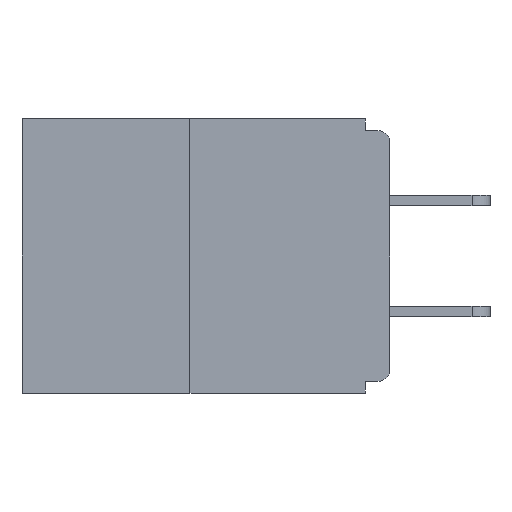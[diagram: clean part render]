
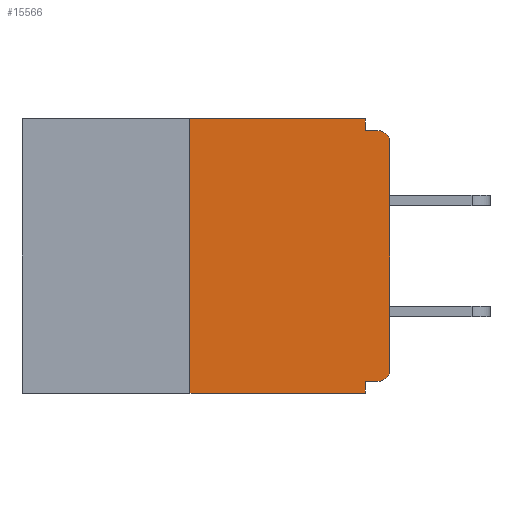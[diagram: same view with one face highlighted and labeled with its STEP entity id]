
A CAD part, left-side view. The second image highlights one B-rep face of the part: STEP entity #15566.
In plain terms, the highlighted planar face has unit normal (-1, 0, 0).
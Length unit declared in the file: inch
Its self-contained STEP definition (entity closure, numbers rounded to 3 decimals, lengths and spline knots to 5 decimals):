
#357 = VERTEX_POINT ( 'NONE', #9742 ) ;
#506 = VECTOR ( 'NONE', #11299, 39.37008 ) ;
#671 = DIRECTION ( 'NONE',  ( 0., 0., 1. ) ) ;
#675 = VECTOR ( 'NONE', #4739, 39.37008 ) ;
#693 = AXIS2_PLACEMENT_3D ( 'NONE', #9688, #7070, #15777 ) ;
#723 = VERTEX_POINT ( 'NONE', #13033 ) ;
#796 = AXIS2_PLACEMENT_3D ( 'NONE', #6944, #5755, #15402 ) ;
#924 = VERTEX_POINT ( 'NONE', #9334 ) ;
#1156 = EDGE_LOOP ( 'NONE', ( #6539, #14464, #13725, #7152, #11252, #13075, #14799, #13834, #2690, #3766 ) ) ;
#1296 = CARTESIAN_POINT ( 'NONE',  ( 0., 0.031, 0. ) ) ;
#1321 = CARTESIAN_POINT ( 'NONE',  ( 0., 0.031, -0.343 ) ) ;
#1667 = DIRECTION ( 'NONE',  ( 0., 0., -1. ) ) ;
#2594 = LINE ( 'NONE', #12889, #14806 ) ;
#2690 = ORIENTED_EDGE ( 'NONE', *, *, #5929, .F. ) ;
#2918 = VERTEX_POINT ( 'NONE', #1321 ) ;
#3150 = DIRECTION ( 'NONE',  ( 0., 0., 1. ) ) ;
#3162 = DIRECTION ( 'NONE',  ( 0., 1., 0. ) ) ;
#3386 = CARTESIAN_POINT ( 'NONE',  ( 0., 0.46, 0. ) ) ;
#3417 = VERTEX_POINT ( 'NONE', #5315 ) ;
#3766 = ORIENTED_EDGE ( 'NONE', *, *, #11858, .F. ) ;
#3894 = CIRCLE ( 'NONE', #693, 0.015 ) ;
#4316 = CARTESIAN_POINT ( 'NONE',  ( 0., 0.031, -0.343 ) ) ;
#4546 = EDGE_CURVE ( 'NONE', #723, #13877, #11496, .T. ) ;
#4739 = DIRECTION ( 'NONE',  ( 0., -1., 0. ) ) ;
#4952 = CIRCLE ( 'NONE', #9415, 0.015 ) ;
#5315 = CARTESIAN_POINT ( 'NONE',  ( 0., 0.031, -0.015 ) ) ;
#5355 = LINE ( 'NONE', #1296, #13733 ) ;
#5410 = EDGE_CURVE ( 'NONE', #14856, #723, #4952, .T. ) ;
#5696 = LINE ( 'NONE', #11544, #9718 ) ;
#5755 = DIRECTION ( 'NONE',  ( 1., 0., 0. ) ) ;
#5929 = EDGE_CURVE ( 'NONE', #3417, #924, #5696, .T. ) ;
#6289 = DIRECTION ( 'NONE',  ( 0., 0., -1. ) ) ;
#6325 = CARTESIAN_POINT ( 'NONE',  ( 0., 0.25, 0. ) ) ;
#6335 = CARTESIAN_POINT ( 'NONE',  ( 0., 0.46, -0.343 ) ) ;
#6442 = DIRECTION ( 'NONE',  ( -1., 0., 0. ) ) ;
#6539 = ORIENTED_EDGE ( 'NONE', *, *, #7238, .F. ) ;
#6703 = CARTESIAN_POINT ( 'NONE',  ( 0., 0., -0.328 ) ) ;
#6776 = CARTESIAN_POINT ( 'NONE',  ( 0., 0., 0. ) ) ;
#6808 = EDGE_CURVE ( 'NONE', #357, #8878, #2594, .T. ) ;
#6944 = CARTESIAN_POINT ( 'NONE',  ( 0., 0.46, 0. ) ) ;
#7070 = DIRECTION ( 'NONE',  ( -1., 0., 0. ) ) ;
#7152 = ORIENTED_EDGE ( 'NONE', *, *, #15572, .F. ) ;
#7238 = EDGE_CURVE ( 'NONE', #8878, #15406, #7567, .T. ) ;
#7567 = LINE ( 'NONE', #3386, #675 ) ;
#7776 = CARTESIAN_POINT ( 'NONE',  ( 0., 0.015, -0.313 ) ) ;
#8025 = DIRECTION ( 'NONE',  ( 0., 0., -1. ) ) ;
#8278 = VECTOR ( 'NONE', #8025, 39.37008 ) ;
#8878 = VERTEX_POINT ( 'NONE', #6325 ) ;
#9004 = CARTESIAN_POINT ( 'NONE',  ( 0., 0.031, -0.328 ) ) ;
#9051 = VERTEX_POINT ( 'NONE', #9004 ) ;
#9243 = FACE_OUTER_BOUND ( 'NONE', #1156, .T. ) ;
#9312 = CARTESIAN_POINT ( 'NONE',  ( 0., 0.031, 0. ) ) ;
#9334 = CARTESIAN_POINT ( 'NONE',  ( 0., 0.015, -0.015 ) ) ;
#9415 = AXIS2_PLACEMENT_3D ( 'NONE', #7776, #6442, #1667 ) ;
#9688 = CARTESIAN_POINT ( 'NONE',  ( 0., 0.015, -0.03 ) ) ;
#9718 = VECTOR ( 'NONE', #15192, 39.37008 ) ;
#9742 = CARTESIAN_POINT ( 'NONE',  ( 0., 0.25, -0.343 ) ) ;
#10521 = VECTOR ( 'NONE', #671, 39.37008 ) ;
#11252 = ORIENTED_EDGE ( 'NONE', *, *, #12905, .F. ) ;
#11299 = DIRECTION ( 'NONE',  ( 0., -1., 0. ) ) ;
#11328 = CARTESIAN_POINT ( 'NONE',  ( 0., 0., -0.03 ) ) ;
#11496 = LINE ( 'NONE', #6776, #10521 ) ;
#11531 = LINE ( 'NONE', #4316, #8278 ) ;
#11544 = CARTESIAN_POINT ( 'NONE',  ( 0., 0., -0.015 ) ) ;
#11667 = PLANE ( 'NONE',  #796 ) ;
#11858 = EDGE_CURVE ( 'NONE', #15406, #3417, #5355, .T. ) ;
#12424 = CARTESIAN_POINT ( 'NONE',  ( 0., 0.015, -0.328 ) ) ;
#12889 = CARTESIAN_POINT ( 'NONE',  ( 0., 0.25, 0. ) ) ;
#12905 = EDGE_CURVE ( 'NONE', #14856, #9051, #13886, .T. ) ;
#13033 = CARTESIAN_POINT ( 'NONE',  ( 0., 0., -0.313 ) ) ;
#13075 = ORIENTED_EDGE ( 'NONE', *, *, #5410, .T. ) ;
#13556 = EDGE_CURVE ( 'NONE', #357, #2918, #15395, .T. ) ;
#13725 = ORIENTED_EDGE ( 'NONE', *, *, #13556, .T. ) ;
#13733 = VECTOR ( 'NONE', #6289, 39.37008 ) ;
#13834 = ORIENTED_EDGE ( 'NONE', *, *, #15175, .T. ) ;
#13877 = VERTEX_POINT ( 'NONE', #11328 ) ;
#13886 = LINE ( 'NONE', #6703, #14068 ) ;
#14068 = VECTOR ( 'NONE', #3162, 39.37008 ) ;
#14464 = ORIENTED_EDGE ( 'NONE', *, *, #6808, .F. ) ;
#14799 = ORIENTED_EDGE ( 'NONE', *, *, #4546, .T. ) ;
#14806 = VECTOR ( 'NONE', #3150, 39.37008 ) ;
#14856 = VERTEX_POINT ( 'NONE', #12424 ) ;
#15175 = EDGE_CURVE ( 'NONE', #13877, #924, #3894, .T. ) ;
#15192 = DIRECTION ( 'NONE',  ( 0., -1., 0. ) ) ;
#15395 = LINE ( 'NONE', #6335, #506 ) ;
#15402 = DIRECTION ( 'NONE',  ( 0., 0., -1. ) ) ;
#15406 = VERTEX_POINT ( 'NONE', #9312 ) ;
#15566 = ADVANCED_FACE ( 'NONE', ( #9243 ), #11667, .F. ) ;
#15572 = EDGE_CURVE ( 'NONE', #9051, #2918, #11531, .T. ) ;
#15777 = DIRECTION ( 'NONE',  ( 0., 0., -1. ) ) ;
